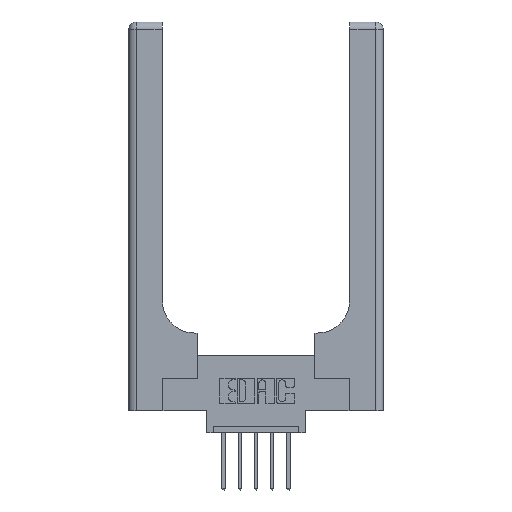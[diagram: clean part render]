
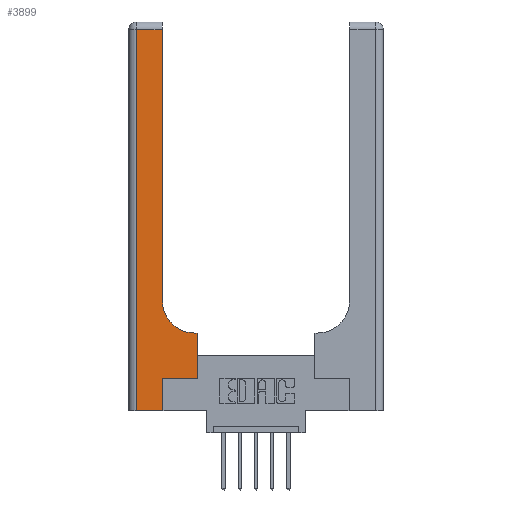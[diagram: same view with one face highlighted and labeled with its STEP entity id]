
A CAD part, top view. The second image highlights one B-rep face of the part: STEP entity #3899.
In plain terms, the highlighted planar face has unit normal (0, 0, 1).
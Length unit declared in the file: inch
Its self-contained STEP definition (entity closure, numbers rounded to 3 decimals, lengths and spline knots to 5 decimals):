
#218 = EDGE_CURVE ( 'NONE', #9813, #5174, #10599, .T. ) ;
#351 = DIRECTION ( 'NONE',  ( 1., 0., 0. ) ) ;
#436 = CARTESIAN_POINT ( 'NONE',  ( 0.265, 0., 0.37 ) ) ;
#560 = CARTESIAN_POINT ( 'NONE',  ( 0.06, 3., 0.37 ) ) ;
#580 = EDGE_LOOP ( 'NONE', ( #9020, #4195, #693, #4022, #13193, #5945, #1056, #3260, #6956 ) ) ;
#693 = ORIENTED_EDGE ( 'NONE', *, *, #8335, .T. ) ;
#694 = CARTESIAN_POINT ( 'NONE',  ( 0.265, 0., 0.37 ) ) ;
#832 = EDGE_CURVE ( 'NONE', #5174, #4108, #13501, .T. ) ;
#1056 = ORIENTED_EDGE ( 'NONE', *, *, #218, .T. ) ;
#1057 = CARTESIAN_POINT ( 'NONE',  ( 0.51, 0.6, 0.37 ) ) ;
#1151 = VECTOR ( 'NONE', #12409, 39.37008 ) ;
#1278 = DIRECTION ( 'NONE',  ( 0., 0., -1. ) ) ;
#1533 = CARTESIAN_POINT ( 'NONE',  ( 0.06, 2.94, 0.37 ) ) ;
#1892 = DIRECTION ( 'NONE',  ( 0., 1., 0. ) ) ;
#2143 = VECTOR ( 'NONE', #351, 39.37008 ) ;
#2498 = VERTEX_POINT ( 'NONE', #10674 ) ;
#2752 = VERTEX_POINT ( 'NONE', #436 ) ;
#2922 = LINE ( 'NONE', #694, #1151 ) ;
#2940 = CARTESIAN_POINT ( 'NONE',  ( 0.26, 3., 0.37 ) ) ;
#3014 = VERTEX_POINT ( 'NONE', #1533 ) ;
#3260 = ORIENTED_EDGE ( 'NONE', *, *, #832, .T. ) ;
#3473 = VECTOR ( 'NONE', #5884, 39.37008 ) ;
#3899 = ADVANCED_FACE ( 'NONE', ( #8643 ), #6598, .F. ) ;
#4022 = ORIENTED_EDGE ( 'NONE', *, *, #13788, .T. ) ;
#4027 = CARTESIAN_POINT ( 'NONE',  ( 0.51, 0.85, 0.37 ) ) ;
#4108 = VERTEX_POINT ( 'NONE', #1057 ) ;
#4195 = ORIENTED_EDGE ( 'NONE', *, *, #12795, .T. ) ;
#4275 = CARTESIAN_POINT ( 'NONE',  ( 0., 2.94, 0.37 ) ) ;
#4509 = AXIS2_PLACEMENT_3D ( 'NONE', #10884, #1278, #9831 ) ;
#4893 = CARTESIAN_POINT ( 'NONE',  ( 0.26, 0.6, 0.37 ) ) ;
#4959 = DIRECTION ( 'NONE',  ( -1., 0., 0. ) ) ;
#5174 = VERTEX_POINT ( 'NONE', #5300 ) ;
#5300 = CARTESIAN_POINT ( 'NONE',  ( 0.528, 0.6, 0.37 ) ) ;
#5728 = VERTEX_POINT ( 'NONE', #6288 ) ;
#5824 = LINE ( 'NONE', #11296, #12761 ) ;
#5884 = DIRECTION ( 'NONE',  ( 0., -1., 0. ) ) ;
#5945 = ORIENTED_EDGE ( 'NONE', *, *, #9259, .T. ) ;
#6288 = CARTESIAN_POINT ( 'NONE',  ( 0.265, 0.25, 0.37 ) ) ;
#6507 = CARTESIAN_POINT ( 'NONE',  ( 0.265, 0.25, 0.37 ) ) ;
#6598 = PLANE ( 'NONE',  #4509 ) ;
#6772 = VECTOR ( 'NONE', #10876, 39.37008 ) ;
#6916 = CARTESIAN_POINT ( 'NONE',  ( 0.528, 0.25, 0.37 ) ) ;
#6956 = ORIENTED_EDGE ( 'NONE', *, *, #9861, .T. ) ;
#7049 = AXIS2_PLACEMENT_3D ( 'NONE', #4027, #9296, #8182 ) ;
#7781 = DIRECTION ( 'NONE',  ( 1., 0., 0. ) ) ;
#8182 = DIRECTION ( 'NONE',  ( 1., 0., 0. ) ) ;
#8335 = EDGE_CURVE ( 'NONE', #3014, #8661, #11285, .T. ) ;
#8625 = LINE ( 'NONE', #6507, #2143 ) ;
#8643 = FACE_OUTER_BOUND ( 'NONE', #580, .T. ) ;
#8661 = VERTEX_POINT ( 'NONE', #12184 ) ;
#9020 = ORIENTED_EDGE ( 'NONE', *, *, #9167, .T. ) ;
#9167 = EDGE_CURVE ( 'NONE', #9480, #2498, #13735, .T. ) ;
#9259 = EDGE_CURVE ( 'NONE', #5728, #9813, #8625, .T. ) ;
#9296 = DIRECTION ( 'NONE',  ( 0., 0., -1. ) ) ;
#9480 = VERTEX_POINT ( 'NONE', #12733 ) ;
#9813 = VERTEX_POINT ( 'NONE', #6916 ) ;
#9831 = DIRECTION ( 'NONE',  ( -1., 0., 0. ) ) ;
#9861 = EDGE_CURVE ( 'NONE', #4108, #9480, #10001, .T. ) ;
#10001 = CIRCLE ( 'NONE', #7049, 0.25 ) ;
#10432 = VECTOR ( 'NONE', #1892, 39.37008 ) ;
#10599 = LINE ( 'NONE', #13810, #6772 ) ;
#10619 = EDGE_CURVE ( 'NONE', #2752, #5728, #2922, .T. ) ;
#10674 = CARTESIAN_POINT ( 'NONE',  ( 0.26, 2.94, 0.37 ) ) ;
#10876 = DIRECTION ( 'NONE',  ( 0., 1., 0. ) ) ;
#10884 = CARTESIAN_POINT ( 'NONE',  ( 0., 3., 0.37 ) ) ;
#11285 = LINE ( 'NONE', #560, #3473 ) ;
#11296 = CARTESIAN_POINT ( 'NONE',  ( 0., 0., 0.37 ) ) ;
#11790 = DIRECTION ( 'NONE',  ( -1., 0., 0. ) ) ;
#12184 = CARTESIAN_POINT ( 'NONE',  ( 0.06, 0., 0.37 ) ) ;
#12409 = DIRECTION ( 'NONE',  ( 0., 1., 0. ) ) ;
#12531 = VECTOR ( 'NONE', #11790, 39.37008 ) ;
#12631 = LINE ( 'NONE', #4275, #12531 ) ;
#12733 = CARTESIAN_POINT ( 'NONE',  ( 0.26, 0.85, 0.37 ) ) ;
#12761 = VECTOR ( 'NONE', #7781, 39.37008 ) ;
#12795 = EDGE_CURVE ( 'NONE', #2498, #3014, #12631, .T. ) ;
#13193 = ORIENTED_EDGE ( 'NONE', *, *, #10619, .T. ) ;
#13381 = VECTOR ( 'NONE', #4959, 39.37008 ) ;
#13501 = LINE ( 'NONE', #4893, #13381 ) ;
#13735 = LINE ( 'NONE', #2940, #10432 ) ;
#13788 = EDGE_CURVE ( 'NONE', #8661, #2752, #5824, .T. ) ;
#13810 = CARTESIAN_POINT ( 'NONE',  ( 0.528, 0.25, 0.37 ) ) ;
